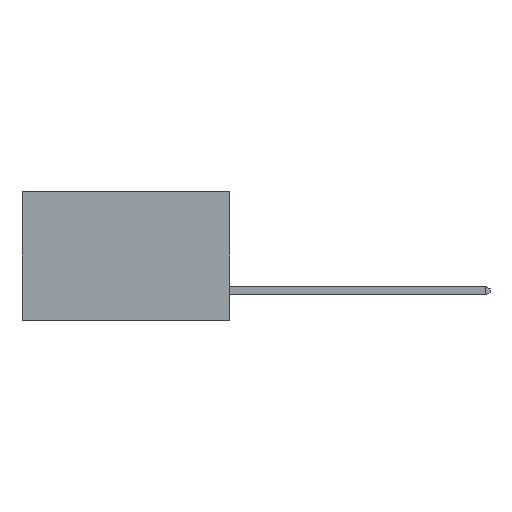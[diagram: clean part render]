
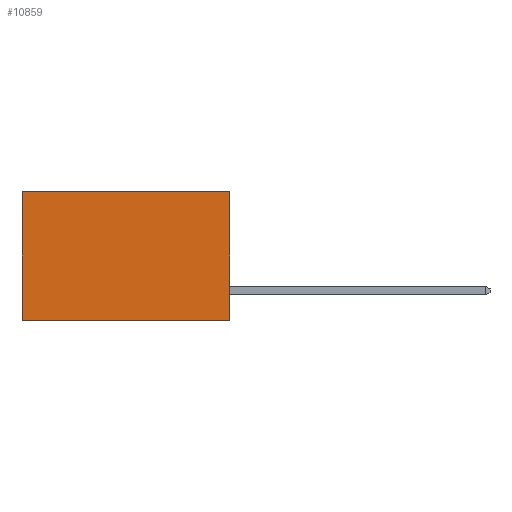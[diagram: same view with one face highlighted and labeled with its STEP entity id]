
A CAD part, left-side view. The second image highlights one B-rep face of the part: STEP entity #10859.
In plain terms, the highlighted planar face has unit normal (-1, 0, 0).
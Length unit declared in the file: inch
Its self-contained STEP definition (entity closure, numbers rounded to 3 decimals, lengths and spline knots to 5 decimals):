
#942 = ORIENTED_EDGE ( 'NONE', *, *, #21913, .F. ) ;
#1870 = VECTOR ( 'NONE', #17678, 39.37008 ) ;
#3348 = CARTESIAN_POINT ( 'NONE',  ( 0.298, 0., -0.37 ) ) ;
#4066 = EDGE_CURVE ( 'NONE', #21957, #15121, #19305, .T. ) ;
#4265 = AXIS2_PLACEMENT_3D ( 'NONE', #15420, #23885, #11092 ) ;
#5074 = VECTOR ( 'NONE', #8424, 39.37008 ) ;
#5634 = CARTESIAN_POINT ( 'NONE',  ( 0.298, 0., 0. ) ) ;
#6230 = CARTESIAN_POINT ( 'NONE',  ( 0.298, 0., -0.37 ) ) ;
#6445 = CARTESIAN_POINT ( 'NONE',  ( 0.298, 0.6, 0. ) ) ;
#7540 = LINE ( 'NONE', #5634, #23997 ) ;
#7704 = CARTESIAN_POINT ( 'NONE',  ( 0.298, 0.6, 0. ) ) ;
#7834 = VERTEX_POINT ( 'NONE', #8857 ) ;
#7949 = CARTESIAN_POINT ( 'NONE',  ( 0.298, 0., 0. ) ) ;
#8424 = DIRECTION ( 'NONE',  ( 0., 1., 0. ) ) ;
#8857 = CARTESIAN_POINT ( 'NONE',  ( 0.298, 0.6, -0.37 ) ) ;
#8871 = PLANE ( 'NONE',  #4265 ) ;
#9077 = CARTESIAN_POINT ( 'NONE',  ( 0.298, 0., 0. ) ) ;
#9238 = FACE_OUTER_BOUND ( 'NONE', #21311, .T. ) ;
#9904 = DIRECTION ( 'NONE',  ( 0., 0., -1. ) ) ;
#10859 = ADVANCED_FACE ( 'NONE', ( #9238 ), #8871, .F. ) ;
#10914 = LINE ( 'NONE', #6230, #5074 ) ;
#11092 = DIRECTION ( 'NONE',  ( 0., 0., -1. ) ) ;
#11868 = EDGE_CURVE ( 'NONE', #26628, #7834, #10914, .T. ) ;
#13618 = LINE ( 'NONE', #7704, #18655 ) ;
#15121 = VERTEX_POINT ( 'NONE', #6445 ) ;
#15420 = CARTESIAN_POINT ( 'NONE',  ( 0.298, 0., 0. ) ) ;
#17678 = DIRECTION ( 'NONE',  ( 0., 1., 0. ) ) ;
#18655 = VECTOR ( 'NONE', #9904, 39.37008 ) ;
#19305 = LINE ( 'NONE', #9077, #1870 ) ;
#21311 = EDGE_LOOP ( 'NONE', ( #24811, #23080, #942, #27188 ) ) ;
#21913 = EDGE_CURVE ( 'NONE', #21957, #26628, #7540, .T. ) ;
#21957 = VERTEX_POINT ( 'NONE', #7949 ) ;
#22923 = DIRECTION ( 'NONE',  ( 0., 0., -1. ) ) ;
#23080 = ORIENTED_EDGE ( 'NONE', *, *, #11868, .F. ) ;
#23885 = DIRECTION ( 'NONE',  ( 1., 0., 0. ) ) ;
#23997 = VECTOR ( 'NONE', #22923, 39.37008 ) ;
#24811 = ORIENTED_EDGE ( 'NONE', *, *, #25978, .T. ) ;
#25978 = EDGE_CURVE ( 'NONE', #15121, #7834, #13618, .T. ) ;
#26628 = VERTEX_POINT ( 'NONE', #3348 ) ;
#27188 = ORIENTED_EDGE ( 'NONE', *, *, #4066, .T. ) ;
